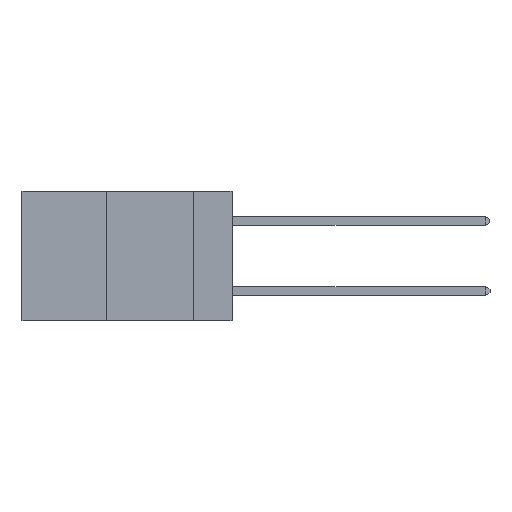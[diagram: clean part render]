
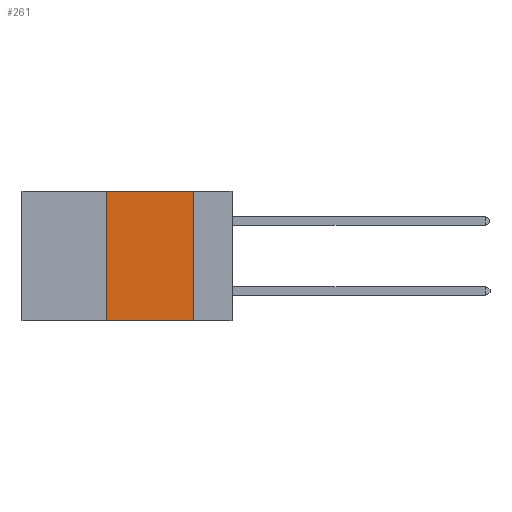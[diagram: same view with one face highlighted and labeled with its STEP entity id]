
A CAD part, left-side view. The second image highlights one B-rep face of the part: STEP entity #261.
In plain terms, the highlighted planar face has unit normal (-1, 0, 0).
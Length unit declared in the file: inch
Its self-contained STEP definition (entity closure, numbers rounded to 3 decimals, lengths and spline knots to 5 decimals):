
#261 = ADVANCED_FACE ( 'NONE', ( #6771 ), #16235, .F. ) ;
#588 = DIRECTION ( 'NONE',  ( 0., 0., -1. ) ) ;
#815 = VECTOR ( 'NONE', #11234, 39.37008 ) ;
#1364 = LINE ( 'NONE', #4531, #815 ) ;
#1515 = CARTESIAN_POINT ( 'NONE',  ( 0., 0.36, 0. ) ) ;
#1857 = CARTESIAN_POINT ( 'NONE',  ( 0., 0.6, 0. ) ) ;
#2236 = EDGE_CURVE ( 'NONE', #2500, #17114, #20250, .T. ) ;
#2314 = EDGE_CURVE ( 'NONE', #2500, #13019, #1364, .T. ) ;
#2473 = CARTESIAN_POINT ( 'NONE',  ( 0., 0.36, 0. ) ) ;
#2500 = VERTEX_POINT ( 'NONE', #5234 ) ;
#3353 = EDGE_CURVE ( 'NONE', #17114, #10349, #17747, .T. ) ;
#4159 = CARTESIAN_POINT ( 'NONE',  ( 0., 0.11, 0. ) ) ;
#4290 = DIRECTION ( 'NONE',  ( 0., 0., 1. ) ) ;
#4531 = CARTESIAN_POINT ( 'NONE',  ( 0., 0.6, -0.37 ) ) ;
#5050 = DIRECTION ( 'NONE',  ( 0., -1., 0. ) ) ;
#5234 = CARTESIAN_POINT ( 'NONE',  ( 0., 0.36, -0.37 ) ) ;
#6412 = EDGE_CURVE ( 'NONE', #10349, #13019, #8451, .T. ) ;
#6771 = FACE_OUTER_BOUND ( 'NONE', #18688, .T. ) ;
#7167 = ORIENTED_EDGE ( 'NONE', *, *, #3353, .F. ) ;
#8360 = VECTOR ( 'NONE', #5050, 39.37008 ) ;
#8451 = LINE ( 'NONE', #4159, #21043 ) ;
#9587 = AXIS2_PLACEMENT_3D ( 'NONE', #1857, #13555, #16462 ) ;
#10349 = VERTEX_POINT ( 'NONE', #11220 ) ;
#11187 = ORIENTED_EDGE ( 'NONE', *, *, #6412, .F. ) ;
#11220 = CARTESIAN_POINT ( 'NONE',  ( 0., 0.11, 0. ) ) ;
#11234 = DIRECTION ( 'NONE',  ( 0., -1., 0. ) ) ;
#11621 = VECTOR ( 'NONE', #4290, 39.37008 ) ;
#11702 = CARTESIAN_POINT ( 'NONE',  ( 0., 0.11, -0.37 ) ) ;
#11712 = ORIENTED_EDGE ( 'NONE', *, *, #2236, .F. ) ;
#13019 = VERTEX_POINT ( 'NONE', #11702 ) ;
#13455 = CARTESIAN_POINT ( 'NONE',  ( 0., 0.6, 0. ) ) ;
#13555 = DIRECTION ( 'NONE',  ( 1., 0., 0. ) ) ;
#16235 = PLANE ( 'NONE',  #9587 ) ;
#16462 = DIRECTION ( 'NONE',  ( 0., 0., -1. ) ) ;
#17114 = VERTEX_POINT ( 'NONE', #1515 ) ;
#17747 = LINE ( 'NONE', #13455, #8360 ) ;
#18688 = EDGE_LOOP ( 'NONE', ( #11187, #7167, #11712, #20331 ) ) ;
#20250 = LINE ( 'NONE', #2473, #11621 ) ;
#20331 = ORIENTED_EDGE ( 'NONE', *, *, #2314, .T. ) ;
#21043 = VECTOR ( 'NONE', #588, 39.37008 ) ;
